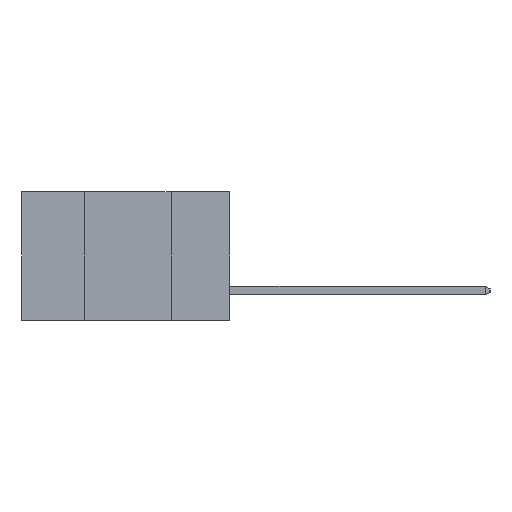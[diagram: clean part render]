
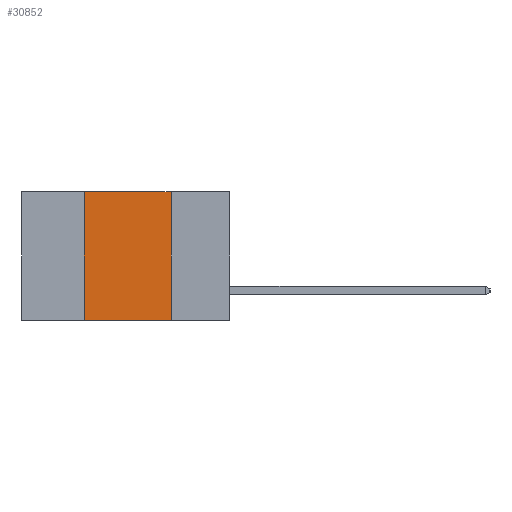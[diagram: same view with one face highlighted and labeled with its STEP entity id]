
A CAD part, left-side view. The second image highlights one B-rep face of the part: STEP entity #30852.
In plain terms, the highlighted planar face has unit normal (-1, 0, 0).
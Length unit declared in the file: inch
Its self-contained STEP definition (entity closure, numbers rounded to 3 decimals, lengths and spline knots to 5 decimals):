
#646 = EDGE_CURVE ( 'NONE', #19065, #17621, #16820, .T. ) ;
#1252 = LINE ( 'NONE', #4630, #20373 ) ;
#1253 = LINE ( 'NONE', #25963, #20376 ) ;
#2139 = DIRECTION ( 'NONE',  ( 0., 0., -1. ) ) ;
#2358 = FACE_OUTER_BOUND ( 'NONE', #9018, .T. ) ;
#2941 = CARTESIAN_POINT ( 'NONE',  ( 0., 0.17, 0. ) ) ;
#4630 = CARTESIAN_POINT ( 'NONE',  ( 0., 0.6, -0.37 ) ) ;
#6141 = LINE ( 'NONE', #2941, #12011 ) ;
#6194 = EDGE_CURVE ( 'NONE', #8072, #19065, #1253, .T. ) ;
#7401 = CARTESIAN_POINT ( 'NONE',  ( 0., 0.17, 0. ) ) ;
#8072 = VERTEX_POINT ( 'NONE', #23587 ) ;
#9018 = EDGE_LOOP ( 'NONE', ( #22414, #17318, #32160, #14589 ) ) ;
#9356 = VECTOR ( 'NONE', #30750, 39.37008 ) ;
#10974 = DIRECTION ( 'NONE',  ( 0., 0., 1. ) ) ;
#12011 = VECTOR ( 'NONE', #25302, 39.37008 ) ;
#12953 = CARTESIAN_POINT ( 'NONE',  ( 0., 0.6, 0. ) ) ;
#14589 = ORIENTED_EDGE ( 'NONE', *, *, #21048, .T. ) ;
#16820 = LINE ( 'NONE', #12953, #9356 ) ;
#17073 = DIRECTION ( 'NONE',  ( 1., 0., 0. ) ) ;
#17318 = ORIENTED_EDGE ( 'NONE', *, *, #646, .F. ) ;
#17621 = VERTEX_POINT ( 'NONE', #7401 ) ;
#19065 = VERTEX_POINT ( 'NONE', #19265 ) ;
#19265 = CARTESIAN_POINT ( 'NONE',  ( 0., 0.42, 0. ) ) ;
#20373 = VECTOR ( 'NONE', #22132, 39.37008 ) ;
#20376 = VECTOR ( 'NONE', #10974, 39.37008 ) ;
#21048 = EDGE_CURVE ( 'NONE', #8072, #21127, #1252, .T. ) ;
#21127 = VERTEX_POINT ( 'NONE', #28444 ) ;
#22132 = DIRECTION ( 'NONE',  ( 0., -1., 0. ) ) ;
#22414 = ORIENTED_EDGE ( 'NONE', *, *, #22850, .F. ) ;
#22850 = EDGE_CURVE ( 'NONE', #17621, #21127, #6141, .T. ) ;
#23587 = CARTESIAN_POINT ( 'NONE',  ( 0., 0.42, -0.37 ) ) ;
#24088 = AXIS2_PLACEMENT_3D ( 'NONE', #32028, #17073, #2139 ) ;
#25302 = DIRECTION ( 'NONE',  ( 0., 0., -1. ) ) ;
#25963 = CARTESIAN_POINT ( 'NONE',  ( 0., 0.42, 0. ) ) ;
#27017 = PLANE ( 'NONE',  #24088 ) ;
#28444 = CARTESIAN_POINT ( 'NONE',  ( 0., 0.17, -0.37 ) ) ;
#30750 = DIRECTION ( 'NONE',  ( 0., -1., 0. ) ) ;
#30852 = ADVANCED_FACE ( 'NONE', ( #2358 ), #27017, .F. ) ;
#32028 = CARTESIAN_POINT ( 'NONE',  ( 0., 0.6, 0. ) ) ;
#32160 = ORIENTED_EDGE ( 'NONE', *, *, #6194, .F. ) ;
